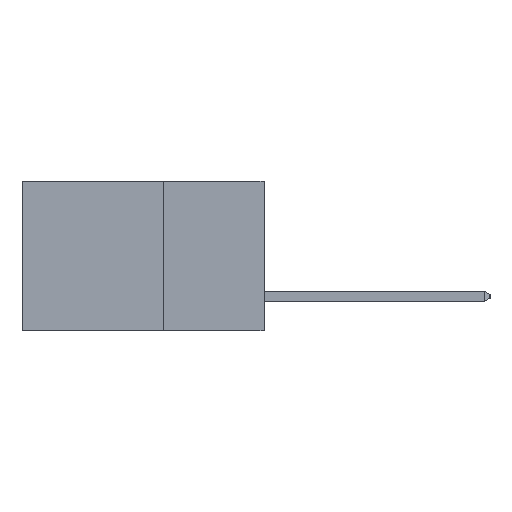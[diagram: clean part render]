
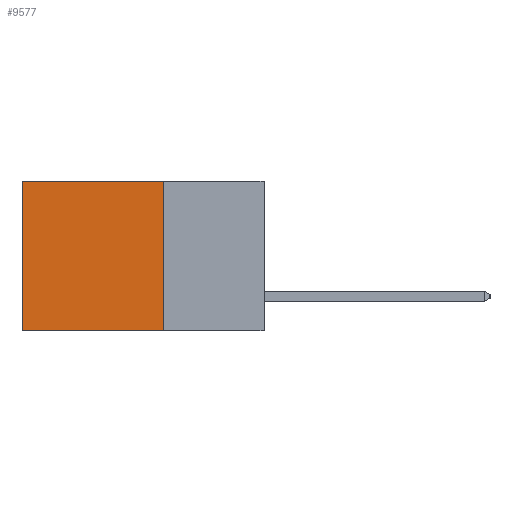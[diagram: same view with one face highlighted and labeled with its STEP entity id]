
A CAD part, left-side view. The second image highlights one B-rep face of the part: STEP entity #9577.
In plain terms, the highlighted planar face has unit normal (-1, 0, 0).
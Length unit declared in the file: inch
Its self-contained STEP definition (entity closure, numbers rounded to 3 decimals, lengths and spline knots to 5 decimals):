
#535 = PLANE ( 'NONE',  #8404 ) ;
#1202 = CARTESIAN_POINT ( 'NONE',  ( 0.2615, 0.25, -0.37 ) ) ;
#1487 = ORIENTED_EDGE ( 'NONE', *, *, #8502, .T. ) ;
#1566 = DIRECTION ( 'NONE',  ( 0., 1., 0. ) ) ;
#1742 = EDGE_CURVE ( 'NONE', #18999, #17791, #20012, .T. ) ;
#3231 = VECTOR ( 'NONE', #5234, 39.37008 ) ;
#4595 = VERTEX_POINT ( 'NONE', #20506 ) ;
#5234 = DIRECTION ( 'NONE',  ( 0., 0., -1. ) ) ;
#5288 = CARTESIAN_POINT ( 'NONE',  ( 0.2615, 0.6, -0.37 ) ) ;
#5583 = CARTESIAN_POINT ( 'NONE',  ( 0.2615, 0.25, -0.37 ) ) ;
#5668 = DIRECTION ( 'NONE',  ( 0., 1., 0. ) ) ;
#6861 = CARTESIAN_POINT ( 'NONE',  ( 0.2615, 0.25, 0. ) ) ;
#8315 = VECTOR ( 'NONE', #5668, 39.37008 ) ;
#8404 = AXIS2_PLACEMENT_3D ( 'NONE', #5583, #13126, #13254 ) ;
#8502 = EDGE_CURVE ( 'NONE', #4595, #17791, #12934, .T. ) ;
#9070 = VERTEX_POINT ( 'NONE', #19562 ) ;
#9577 = ADVANCED_FACE ( 'NONE', ( #18330 ), #535, .F. ) ;
#10781 = LINE ( 'NONE', #19627, #19533 ) ;
#11020 = CARTESIAN_POINT ( 'NONE',  ( 0.2615, 0.25, -0.37 ) ) ;
#11052 = EDGE_CURVE ( 'NONE', #9070, #4595, #22121, .T. ) ;
#12434 = EDGE_LOOP ( 'NONE', ( #1487, #19443, #14950, #16102 ) ) ;
#12934 = LINE ( 'NONE', #5288, #3231 ) ;
#13126 = DIRECTION ( 'NONE',  ( 1., 0., 0. ) ) ;
#13254 = DIRECTION ( 'NONE',  ( 0., 0., -1. ) ) ;
#14391 = VECTOR ( 'NONE', #1566, 39.37008 ) ;
#14776 = CARTESIAN_POINT ( 'NONE',  ( 0.2615, 0.6, -0.37 ) ) ;
#14950 = ORIENTED_EDGE ( 'NONE', *, *, #15094, .F. ) ;
#15094 = EDGE_CURVE ( 'NONE', #9070, #18999, #10781, .T. ) ;
#16102 = ORIENTED_EDGE ( 'NONE', *, *, #11052, .T. ) ;
#17791 = VERTEX_POINT ( 'NONE', #14776 ) ;
#17992 = DIRECTION ( 'NONE',  ( 0., 0., -1. ) ) ;
#18330 = FACE_OUTER_BOUND ( 'NONE', #12434, .T. ) ;
#18999 = VERTEX_POINT ( 'NONE', #11020 ) ;
#19443 = ORIENTED_EDGE ( 'NONE', *, *, #1742, .F. ) ;
#19533 = VECTOR ( 'NONE', #17992, 39.37008 ) ;
#19562 = CARTESIAN_POINT ( 'NONE',  ( 0.2615, 0.25, 0. ) ) ;
#19627 = CARTESIAN_POINT ( 'NONE',  ( 0.2615, 0.25, -0.37 ) ) ;
#20012 = LINE ( 'NONE', #1202, #14391 ) ;
#20506 = CARTESIAN_POINT ( 'NONE',  ( 0.2615, 0.6, 0. ) ) ;
#22121 = LINE ( 'NONE', #6861, #8315 ) ;
